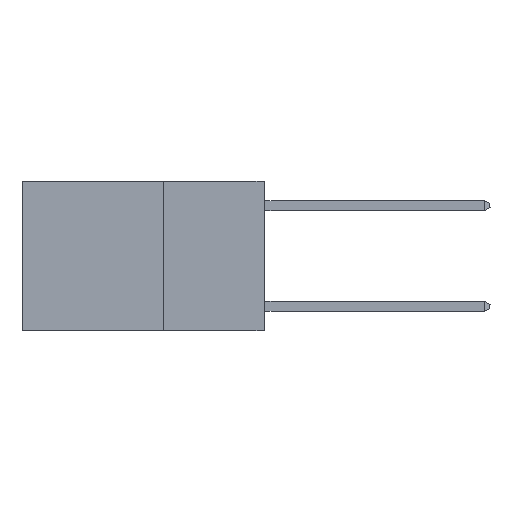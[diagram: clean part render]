
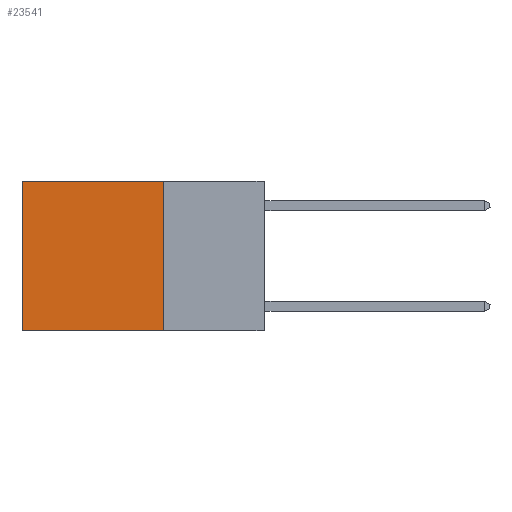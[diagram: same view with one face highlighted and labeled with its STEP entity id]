
A CAD part, left-side view. The second image highlights one B-rep face of the part: STEP entity #23541.
In plain terms, the highlighted planar face has unit normal (-1, 0, 0).
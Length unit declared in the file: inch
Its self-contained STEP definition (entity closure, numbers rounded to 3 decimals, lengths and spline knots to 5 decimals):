
#65 = EDGE_CURVE ( 'NONE', #13111, #22274, #5049, .T. ) ;
#1793 = ORIENTED_EDGE ( 'NONE', *, *, #4109, .T. ) ;
#2391 = EDGE_LOOP ( 'NONE', ( #1793, #16224, #15009, #22160 ) ) ;
#4109 = EDGE_CURVE ( 'NONE', #5008, #22274, #8810, .T. ) ;
#5008 = VERTEX_POINT ( 'NONE', #22947 ) ;
#5049 = LINE ( 'NONE', #7415, #9642 ) ;
#5373 = CARTESIAN_POINT ( 'NONE',  ( 0.2625, 0.25, -0.37 ) ) ;
#6031 = VERTEX_POINT ( 'NONE', #27930 ) ;
#6241 = LINE ( 'NONE', #18642, #6592 ) ;
#6422 = DIRECTION ( 'NONE',  ( 0., 0., -1. ) ) ;
#6592 = VECTOR ( 'NONE', #11189, 39.37008 ) ;
#7205 = VECTOR ( 'NONE', #6422, 39.37008 ) ;
#7228 = EDGE_CURVE ( 'NONE', #6031, #5008, #6241, .T. ) ;
#7415 = CARTESIAN_POINT ( 'NONE',  ( 0.2625, 0.25, -0.37 ) ) ;
#8810 = LINE ( 'NONE', #18509, #7205 ) ;
#9642 = VECTOR ( 'NONE', #12018, 39.37008 ) ;
#11189 = DIRECTION ( 'NONE',  ( 0., 1., 0. ) ) ;
#11446 = CARTESIAN_POINT ( 'NONE',  ( 0.2625, 0.25, 0. ) ) ;
#12018 = DIRECTION ( 'NONE',  ( 0., 1., 0. ) ) ;
#12330 = AXIS2_PLACEMENT_3D ( 'NONE', #11446, #13211, #15597 ) ;
#12384 = CARTESIAN_POINT ( 'NONE',  ( 0.2625, 0.25, 0. ) ) ;
#12707 = DIRECTION ( 'NONE',  ( 0., 0., -1. ) ) ;
#13111 = VERTEX_POINT ( 'NONE', #5373 ) ;
#13211 = DIRECTION ( 'NONE',  ( 1., 0., 0. ) ) ;
#15009 = ORIENTED_EDGE ( 'NONE', *, *, #26960, .F. ) ;
#15597 = DIRECTION ( 'NONE',  ( 0., 0., -1. ) ) ;
#16224 = ORIENTED_EDGE ( 'NONE', *, *, #65, .F. ) ;
#18509 = CARTESIAN_POINT ( 'NONE',  ( 0.2625, 0.6, 0. ) ) ;
#18642 = CARTESIAN_POINT ( 'NONE',  ( 0.2625, 0.25, 0. ) ) ;
#19883 = LINE ( 'NONE', #12384, #19896 ) ;
#19896 = VECTOR ( 'NONE', #12707, 39.37008 ) ;
#22160 = ORIENTED_EDGE ( 'NONE', *, *, #7228, .T. ) ;
#22274 = VERTEX_POINT ( 'NONE', #24616 ) ;
#22947 = CARTESIAN_POINT ( 'NONE',  ( 0.2625, 0.6, 0. ) ) ;
#23541 = ADVANCED_FACE ( 'NONE', ( #27891 ), #25640, .F. ) ;
#24616 = CARTESIAN_POINT ( 'NONE',  ( 0.2625, 0.6, -0.37 ) ) ;
#25640 = PLANE ( 'NONE',  #12330 ) ;
#26960 = EDGE_CURVE ( 'NONE', #6031, #13111, #19883, .T. ) ;
#27891 = FACE_OUTER_BOUND ( 'NONE', #2391, .T. ) ;
#27930 = CARTESIAN_POINT ( 'NONE',  ( 0.2625, 0.25, 0. ) ) ;
